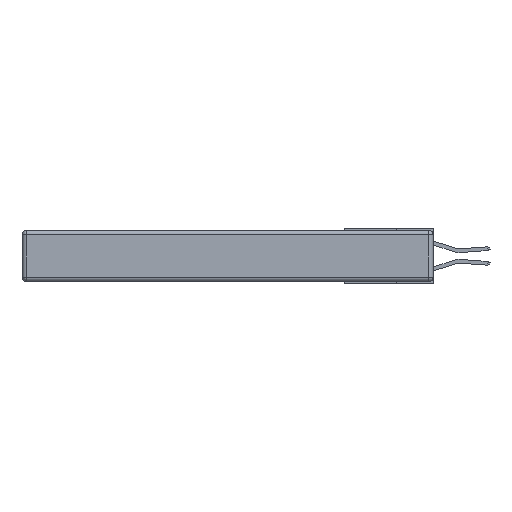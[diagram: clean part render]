
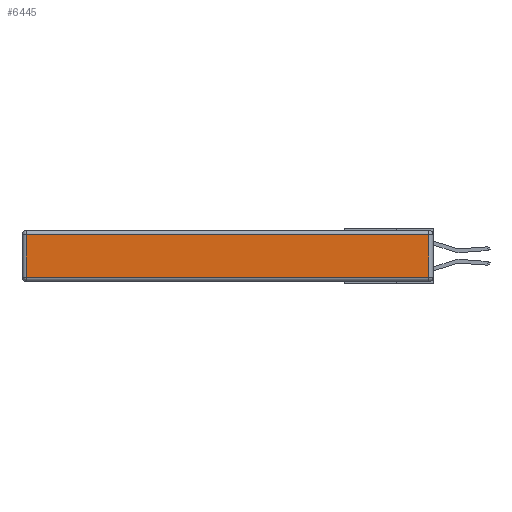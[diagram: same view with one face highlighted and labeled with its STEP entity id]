
A CAD part, left-side view. The second image highlights one B-rep face of the part: STEP entity #6445.
In plain terms, the highlighted planar face has unit normal (-1, 0, 0).
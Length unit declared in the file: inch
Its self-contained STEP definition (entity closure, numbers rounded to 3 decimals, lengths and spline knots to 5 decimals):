
#432 = DIRECTION ( 'NONE',  ( 0., 0., -1. ) ) ;
#497 = VECTOR ( 'NONE', #432, 39.37008 ) ;
#567 = AXIS2_PLACEMENT_3D ( 'NONE', #15729, #12882, #10238 ) ;
#1533 = VECTOR ( 'NONE', #9143, 39.37008 ) ;
#1812 = DIRECTION ( 'NONE',  ( 0., 1., 0. ) ) ;
#3300 = CARTESIAN_POINT ( 'NONE',  ( 0., 2.72, -0.03 ) ) ;
#3883 = EDGE_CURVE ( 'NONE', #8588, #4615, #17520, .T. ) ;
#4473 = ORIENTED_EDGE ( 'NONE', *, *, #9690, .T. ) ;
#4533 = CARTESIAN_POINT ( 'NONE',  ( 0., 2.75, -0.03 ) ) ;
#4615 = VERTEX_POINT ( 'NONE', #3300 ) ;
#4694 = PLANE ( 'NONE',  #567 ) ;
#5873 = EDGE_CURVE ( 'NONE', #4615, #8428, #10882, .T. ) ;
#6445 = ADVANCED_FACE ( 'NONE', ( #7412 ), #4694, .T. ) ;
#7053 = VECTOR ( 'NONE', #1812, 39.37008 ) ;
#7412 = FACE_OUTER_BOUND ( 'NONE', #11895, .T. ) ;
#7728 = VECTOR ( 'NONE', #15540, 39.37008 ) ;
#8428 = VERTEX_POINT ( 'NONE', #12348 ) ;
#8588 = VERTEX_POINT ( 'NONE', #16882 ) ;
#9143 = DIRECTION ( 'NONE',  ( 0., -1., 0. ) ) ;
#9210 = VERTEX_POINT ( 'NONE', #12373 ) ;
#9690 = EDGE_CURVE ( 'NONE', #8428, #9210, #17632, .T. ) ;
#9982 = CARTESIAN_POINT ( 'NONE',  ( 0., 0.03, -0.343 ) ) ;
#10238 = DIRECTION ( 'NONE',  ( 0., 0., 1. ) ) ;
#10549 = EDGE_CURVE ( 'NONE', #9210, #8588, #13162, .T. ) ;
#10657 = ORIENTED_EDGE ( 'NONE', *, *, #10549, .T. ) ;
#10882 = LINE ( 'NONE', #12902, #497 ) ;
#11895 = EDGE_LOOP ( 'NONE', ( #4473, #10657, #12953, #12741 ) ) ;
#12348 = CARTESIAN_POINT ( 'NONE',  ( 0., 2.72, -0.313 ) ) ;
#12373 = CARTESIAN_POINT ( 'NONE',  ( 0., 0.03, -0.313 ) ) ;
#12741 = ORIENTED_EDGE ( 'NONE', *, *, #5873, .T. ) ;
#12882 = DIRECTION ( 'NONE',  ( -1., 0., 0. ) ) ;
#12902 = CARTESIAN_POINT ( 'NONE',  ( 0., 2.72, -0.343 ) ) ;
#12953 = ORIENTED_EDGE ( 'NONE', *, *, #3883, .T. ) ;
#13162 = LINE ( 'NONE', #9982, #7728 ) ;
#15540 = DIRECTION ( 'NONE',  ( 0., 0., 1. ) ) ;
#15729 = CARTESIAN_POINT ( 'NONE',  ( 0., 0., -0.343 ) ) ;
#16140 = CARTESIAN_POINT ( 'NONE',  ( 0., 0., -0.313 ) ) ;
#16882 = CARTESIAN_POINT ( 'NONE',  ( 0., 0.03, -0.03 ) ) ;
#17520 = LINE ( 'NONE', #4533, #7053 ) ;
#17632 = LINE ( 'NONE', #16140, #1533 ) ;
